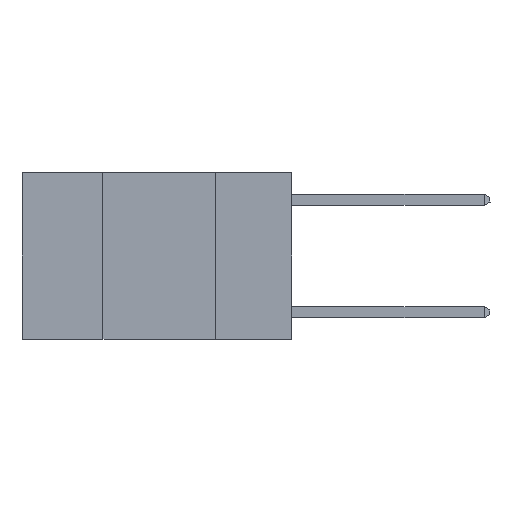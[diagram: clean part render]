
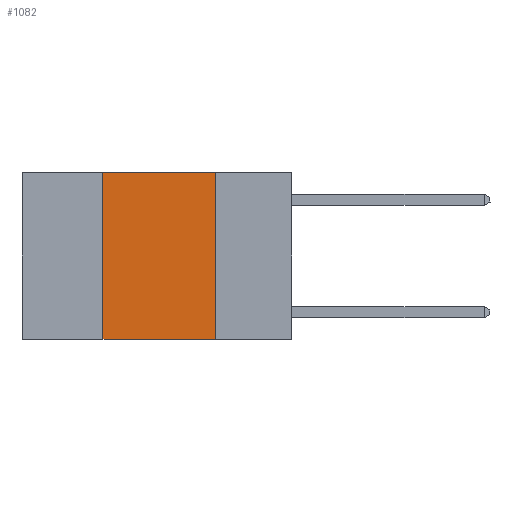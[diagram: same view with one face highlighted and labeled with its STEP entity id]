
A CAD part, left-side view. The second image highlights one B-rep face of the part: STEP entity #1082.
In plain terms, the highlighted planar face has unit normal (-1, 0, 0).
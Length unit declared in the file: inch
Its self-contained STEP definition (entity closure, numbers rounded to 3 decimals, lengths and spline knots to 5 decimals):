
#258 = VECTOR ( 'NONE', #10381, 39.37008 ) ;
#271 = EDGE_CURVE ( 'NONE', #6411, #5667, #6045, .T. ) ;
#493 = LINE ( 'NONE', #10363, #258 ) ;
#1082 = ADVANCED_FACE ( 'NONE', ( #10284 ), #8195, .F. ) ;
#1110 = ORIENTED_EDGE ( 'NONE', *, *, #2570, .T. ) ;
#1486 = EDGE_CURVE ( 'NONE', #5667, #3563, #493, .T. ) ;
#2087 = DIRECTION ( 'NONE',  ( 0., 0., 1. ) ) ;
#2218 = EDGE_LOOP ( 'NONE', ( #2825, #4267, #4561, #1110 ) ) ;
#2551 = CARTESIAN_POINT ( 'NONE',  ( 0., 0.17, 0. ) ) ;
#2562 = CARTESIAN_POINT ( 'NONE',  ( 0., 0.42, -0.37 ) ) ;
#2570 = EDGE_CURVE ( 'NONE', #6411, #8596, #4502, .T. ) ;
#2825 = ORIENTED_EDGE ( 'NONE', *, *, #2891, .F. ) ;
#2891 = EDGE_CURVE ( 'NONE', #3563, #8596, #8735, .T. ) ;
#3563 = VERTEX_POINT ( 'NONE', #2551 ) ;
#4244 = VECTOR ( 'NONE', #7439, 39.37008 ) ;
#4267 = ORIENTED_EDGE ( 'NONE', *, *, #1486, .F. ) ;
#4502 = LINE ( 'NONE', #7503, #4244 ) ;
#4561 = ORIENTED_EDGE ( 'NONE', *, *, #271, .F. ) ;
#5667 = VERTEX_POINT ( 'NONE', #9329 ) ;
#5697 = CARTESIAN_POINT ( 'NONE',  ( 0., 0.17, 0. ) ) ;
#5745 = DIRECTION ( 'NONE',  ( 0., 0., -1. ) ) ;
#5833 = VECTOR ( 'NONE', #5745, 39.37008 ) ;
#6045 = LINE ( 'NONE', #8536, #6259 ) ;
#6259 = VECTOR ( 'NONE', #2087, 39.37008 ) ;
#6411 = VERTEX_POINT ( 'NONE', #2562 ) ;
#7439 = DIRECTION ( 'NONE',  ( 0., -1., 0. ) ) ;
#7503 = CARTESIAN_POINT ( 'NONE',  ( 0., 0.6, -0.37 ) ) ;
#8116 = DIRECTION ( 'NONE',  ( 0., 0., -1. ) ) ;
#8132 = DIRECTION ( 'NONE',  ( 1., 0., 0. ) ) ;
#8156 = CARTESIAN_POINT ( 'NONE',  ( 0., 0.6, 0. ) ) ;
#8195 = PLANE ( 'NONE',  #8282 ) ;
#8282 = AXIS2_PLACEMENT_3D ( 'NONE', #8156, #8132, #8116 ) ;
#8536 = CARTESIAN_POINT ( 'NONE',  ( 0., 0.42, 0. ) ) ;
#8596 = VERTEX_POINT ( 'NONE', #10531 ) ;
#8735 = LINE ( 'NONE', #5697, #5833 ) ;
#9329 = CARTESIAN_POINT ( 'NONE',  ( 0., 0.42, 0. ) ) ;
#10284 = FACE_OUTER_BOUND ( 'NONE', #2218, .T. ) ;
#10363 = CARTESIAN_POINT ( 'NONE',  ( 0., 0.6, 0. ) ) ;
#10381 = DIRECTION ( 'NONE',  ( 0., -1., 0. ) ) ;
#10531 = CARTESIAN_POINT ( 'NONE',  ( 0., 0.17, -0.37 ) ) ;
